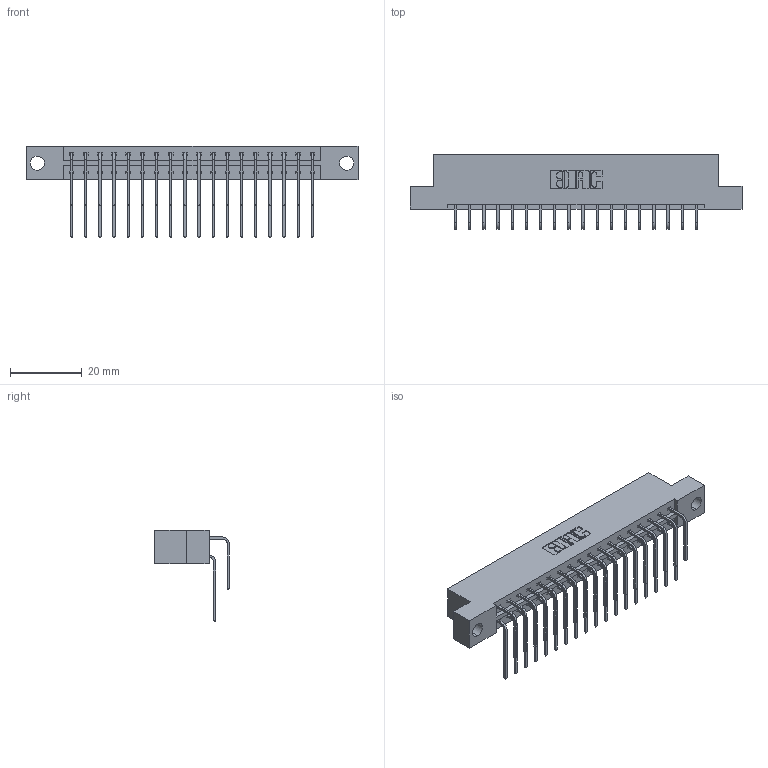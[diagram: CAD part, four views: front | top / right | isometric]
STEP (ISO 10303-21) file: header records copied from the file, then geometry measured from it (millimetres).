
FILE_DESCRIPTION (( 'STEP AP203' ), '1' );
FILE_NAME ('833-036-559-204.STEP', '2020-06-03T04:13:21', ( '' ), ( '' ), 'SwSTEP 2.0', 'SolidWorks 2020', '' );
FILE_SCHEMA (( 'CONFIG_CONTROL_DESIGN' ));
Length unit declared in the file: inch
Products named in the file (4): 833-036-559-204; 345-292-001_559 Tail - 2; 345-292-001_558 559 Tail - 1; 833 Part_Flush - .156 Dia - TH
Assembly tree (37 placements, depth 2):
  833-036-559-204
    833 Part_Flush - .156 Dia - TH
    345-292-001_558 559 Tail - 1  x18
    345-292-001_559 Tail - 2  x18
Bounding box: 92.86 x 20.9 x 25.53 mm (x, y, z)
Volume: 9376.1 mm3; surface area: 11660.9 mm2
Topology: 37 solids, 37 shells, 2058 faces, 6107 edges, 4022 vertices
Faces by surface type: plane 1438, cylinder 620
Entity records: 16471 total; most frequent: CARTESIAN_POINT 2809, ORIENTED_EDGE 2694, DIRECTION 2423, EDGE_CURVE 1347, LINE 1179, VECTOR 1179, VERTEX_POINT 894, AXIS2_PLACEMENT_3D 622
